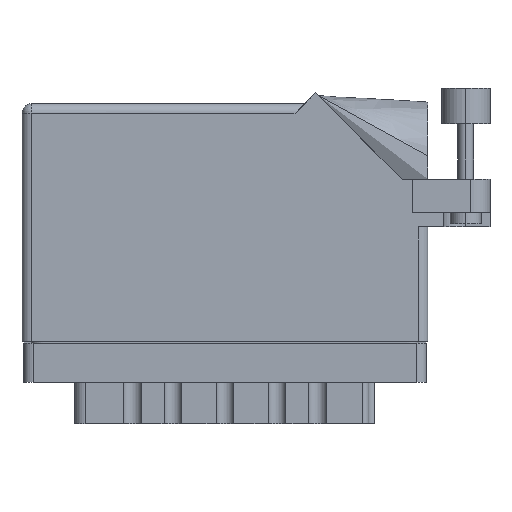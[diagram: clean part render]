
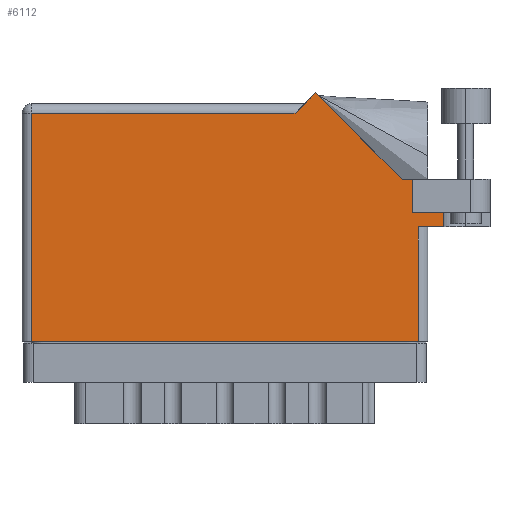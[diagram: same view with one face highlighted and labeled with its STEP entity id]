
A CAD part, front view. The second image highlights one B-rep face of the part: STEP entity #6112.
In plain terms, the highlighted face is planar.
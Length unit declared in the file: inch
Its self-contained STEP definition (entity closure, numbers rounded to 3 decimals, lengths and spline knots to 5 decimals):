
#3099 = VERTEX_POINT ( 'NONE', #34304 ) ;
#3102 = CARTESIAN_POINT ( 'NONE',  ( 2.612, 0.737, 0. ) ) ;
#3352 = DIRECTION ( 'NONE',  ( 1., 0., 0. ) ) ;
#3712 = ORIENTED_EDGE ( 'NONE', *, *, #7377, .T. ) ;
#4376 = LINE ( 'NONE', #19767, #7170 ) ;
#5893 = VERTEX_POINT ( 'NONE', #25286 ) ;
#6027 = CARTESIAN_POINT ( 'NONE',  ( 2.55, 0.737, 0. ) ) ;
#6112 = ADVANCED_FACE ( 'NONE', ( #17608 ), #17097, .F. ) ;
#7170 = VECTOR ( 'NONE', #35166, 39.37008 ) ;
#7377 = EDGE_CURVE ( 'NONE', #38392, #33975, #13141, .T. ) ;
#7496 = VECTOR ( 'NONE', #26926, 39.37008 ) ;
#7833 = CARTESIAN_POINT ( 'NONE',  ( 2.512, 0.831, 0. ) ) ;
#8747 = ORIENTED_EDGE ( 'NONE', *, *, #37239, .T. ) ;
#8965 = VECTOR ( 'NONE', #38374, 39.37008 ) ;
#9235 = CARTESIAN_POINT ( 'NONE',  ( 2.55, 0., 0. ) ) ;
#9388 = DIRECTION ( 'NONE',  ( -1., 0., 0. ) ) ;
#10099 = ORIENTED_EDGE ( 'NONE', *, *, #16032, .T. ) ;
#10156 = LINE ( 'NONE', #49241, #32688 ) ;
#10311 = CARTESIAN_POINT ( 'NONE',  ( 2.512, 0.831, 0. ) ) ;
#11086 = EDGE_CURVE ( 'NONE', #11904, #11537, #41594, .T. ) ;
#11537 = VERTEX_POINT ( 'NONE', #33474 ) ;
#11904 = VERTEX_POINT ( 'NONE', #21779 ) ;
#12384 = ORIENTED_EDGE ( 'NONE', *, *, #27946, .F. ) ;
#12490 = EDGE_LOOP ( 'NONE', ( #48373, #40640, #8747, #12384, #33863, #10099, #41177, #17795, #21885, #29077, #3712 ) ) ;
#12811 = VECTOR ( 'NONE', #27555, 39.37008 ) ;
#13141 = LINE ( 'NONE', #20216, #22929 ) ;
#13170 = CARTESIAN_POINT ( 'NONE',  ( 3.012, 1.044, 0. ) ) ;
#13565 = CARTESIAN_POINT ( 'NONE',  ( 0., 1.53, 0. ) ) ;
#13986 = CARTESIAN_POINT ( 'NONE',  ( 0., 0., 0. ) ) ;
#14081 = LINE ( 'NONE', #30207, #7496 ) ;
#15078 = EDGE_CURVE ( 'NONE', #24223, #3099, #14081, .T. ) ;
#15965 = CARTESIAN_POINT ( 'NONE',  ( 1.819, 1.53, 0. ) ) ;
#16032 = EDGE_CURVE ( 'NONE', #11904, #5893, #38859, .T. ) ;
#17097 = PLANE ( 'NONE',  #32516 ) ;
#17384 = DIRECTION ( 'NONE',  ( 0., 1., 0. ) ) ;
#17608 = FACE_OUTER_BOUND ( 'NONE', #12490, .T. ) ;
#17795 = ORIENTED_EDGE ( 'NONE', *, *, #15078, .T. ) ;
#18384 = LINE ( 'NONE', #6027, #46996 ) ;
#19330 = VERTEX_POINT ( 'NONE', #9235 ) ;
#19767 = CARTESIAN_POINT ( 'NONE',  ( 2.7135, 1.16177, 0. ) ) ;
#20216 = CARTESIAN_POINT ( 'NONE',  ( 0.062, 0., 0. ) ) ;
#20360 = CARTESIAN_POINT ( 'NONE',  ( 2.44642, 1.044, 0. ) ) ;
#21779 = CARTESIAN_POINT ( 'NONE',  ( 2.512, 0.831, 0. ) ) ;
#21885 = ORIENTED_EDGE ( 'NONE', *, *, #28044, .T. ) ;
#22394 = DIRECTION ( 'NONE',  ( 1., 0., 0. ) ) ;
#22929 = VECTOR ( 'NONE', #35893, 39.37008 ) ;
#24223 = VERTEX_POINT ( 'NONE', #20360 ) ;
#24639 = VERTEX_POINT ( 'NONE', #35974 ) ;
#25043 = LINE ( 'NONE', #3102, #40876 ) ;
#25286 = CARTESIAN_POINT ( 'NONE',  ( 2.512, 1.044, 0. ) ) ;
#25938 = VECTOR ( 'NONE', #9388, 39.37008 ) ;
#26926 = DIRECTION ( 'NONE',  ( -0.707, 0.707, 0. ) ) ;
#27354 = VERTEX_POINT ( 'NONE', #29150 ) ;
#27555 = DIRECTION ( 'NONE',  ( -0.707, -0.707, 0. ) ) ;
#27946 = EDGE_CURVE ( 'NONE', #11537, #31261, #4376, .T. ) ;
#28044 = EDGE_CURVE ( 'NONE', #3099, #24639, #31110, .T. ) ;
#28942 = DIRECTION ( 'NONE',  ( 0., 0., -1. ) ) ;
#29063 = EDGE_CURVE ( 'NONE', #33975, #19330, #29613, .T. ) ;
#29077 = ORIENTED_EDGE ( 'NONE', *, *, #49454, .T. ) ;
#29150 = CARTESIAN_POINT ( 'NONE',  ( 2.55, 0.737, 0. ) ) ;
#29296 = EDGE_CURVE ( 'NONE', #5893, #24223, #39682, .T. ) ;
#29613 = LINE ( 'NONE', #13986, #39653 ) ;
#29839 = DIRECTION ( 'NONE',  ( 1., 0., 0. ) ) ;
#30207 = CARTESIAN_POINT ( 'NONE',  ( 2.44642, 1.044, 0. ) ) ;
#31110 = LINE ( 'NONE', #15965, #12811 ) ;
#31261 = VERTEX_POINT ( 'NONE', #34634 ) ;
#32516 = AXIS2_PLACEMENT_3D ( 'NONE', #13565, #28942, #44367 ) ;
#32688 = VECTOR ( 'NONE', #40940, 39.37008 ) ;
#33474 = CARTESIAN_POINT ( 'NONE',  ( 2.7135, 0.831, 0. ) ) ;
#33843 = CARTESIAN_POINT ( 'NONE',  ( 0.062, 0., 0. ) ) ;
#33863 = ORIENTED_EDGE ( 'NONE', *, *, #11086, .F. ) ;
#33975 = VERTEX_POINT ( 'NONE', #33843 ) ;
#34304 = CARTESIAN_POINT ( 'NONE',  ( 1.88971, 1.60071, 0. ) ) ;
#34634 = CARTESIAN_POINT ( 'NONE',  ( 2.7135, 0.737, 0. ) ) ;
#35166 = DIRECTION ( 'NONE',  ( 0., -1., 0. ) ) ;
#35893 = DIRECTION ( 'NONE',  ( 0., -1., 0. ) ) ;
#35974 = CARTESIAN_POINT ( 'NONE',  ( 1.757, 1.468, 0. ) ) ;
#37239 = EDGE_CURVE ( 'NONE', #27354, #31261, #25043, .T. ) ;
#38374 = DIRECTION ( 'NONE',  ( 0., 1., 0. ) ) ;
#38392 = VERTEX_POINT ( 'NONE', #39999 ) ;
#38859 = LINE ( 'NONE', #7833, #8965 ) ;
#39653 = VECTOR ( 'NONE', #3352, 39.37008 ) ;
#39682 = LINE ( 'NONE', #13170, #25938 ) ;
#39999 = CARTESIAN_POINT ( 'NONE',  ( 0.062, 1.468, 0. ) ) ;
#40640 = ORIENTED_EDGE ( 'NONE', *, *, #45453, .T. ) ;
#40876 = VECTOR ( 'NONE', #29839, 39.37008 ) ;
#40940 = DIRECTION ( 'NONE',  ( -1., 0., 0. ) ) ;
#41177 = ORIENTED_EDGE ( 'NONE', *, *, #29296, .T. ) ;
#41594 = LINE ( 'NONE', #10311, #43331 ) ;
#43331 = VECTOR ( 'NONE', #22394, 39.37008 ) ;
#44367 = DIRECTION ( 'NONE',  ( -1., 0., 0. ) ) ;
#45453 = EDGE_CURVE ( 'NONE', #19330, #27354, #18384, .T. ) ;
#46996 = VECTOR ( 'NONE', #17384, 39.37008 ) ;
#48373 = ORIENTED_EDGE ( 'NONE', *, *, #29063, .T. ) ;
#49241 = CARTESIAN_POINT ( 'NONE',  ( 0., 1.468, 0. ) ) ;
#49454 = EDGE_CURVE ( 'NONE', #24639, #38392, #10156, .T. ) ;
